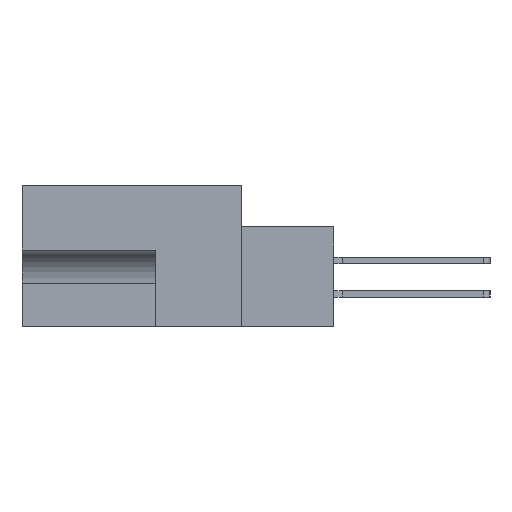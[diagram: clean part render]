
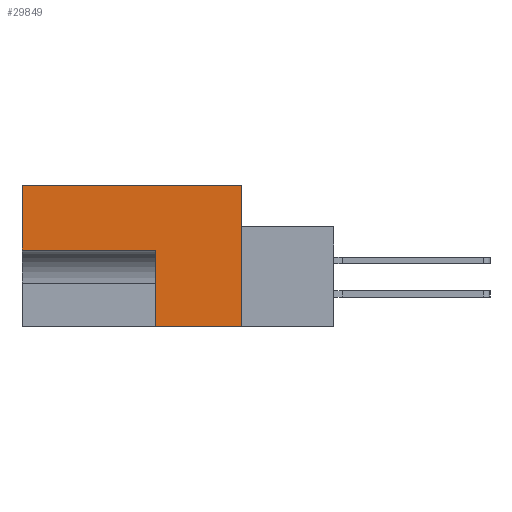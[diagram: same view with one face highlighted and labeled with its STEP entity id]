
A CAD part, left-side view. The second image highlights one B-rep face of the part: STEP entity #29849.
In plain terms, the highlighted planar face has unit normal (-1, 0, 0).
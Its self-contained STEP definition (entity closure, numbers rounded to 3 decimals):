
#51 = VERTEX_POINT ( 'NONE', #46277 ) ;
#1317 = DIRECTION ( 'NONE',  ( 1., 0., 0. ) ) ;
#1569 = ORIENTED_EDGE ( 'NONE', *, *, #10130, .F. ) ;
#1701 = DIRECTION ( 'NONE',  ( 0., 0., -1. ) ) ;
#2221 = ORIENTED_EDGE ( 'NONE', *, *, #9376, .F. ) ;
#2497 = AXIS2_PLACEMENT_3D ( 'NONE', #43975, #1317, #15414 ) ;
#2968 = VERTEX_POINT ( 'NONE', #28718 ) ;
#4047 = EDGE_CURVE ( 'NONE', #51, #22606, #5788, .T. ) ;
#5521 = EDGE_CURVE ( 'NONE', #15819, #34559, #16864, .T. ) ;
#5788 = LINE ( 'NONE', #9477, #11433 ) ;
#6238 = EDGE_LOOP ( 'NONE', ( #42021, #45216, #1569, #29505, #16491, #2221 ) ) ;
#6247 = VECTOR ( 'NONE', #1701, 1000. ) ;
#6517 = CARTESIAN_POINT ( 'NONE',  ( 0., 8.255, -13.487 ) ) ;
#7277 = FACE_OUTER_BOUND ( 'NONE', #6238, .T. ) ;
#9376 = EDGE_CURVE ( 'NONE', #30089, #51, #42847, .T. ) ;
#9457 = EDGE_CURVE ( 'NONE', #34559, #30089, #16005, .T. ) ;
#9477 = CARTESIAN_POINT ( 'NONE',  ( 0., 8.255, -6.172 ) ) ;
#9478 = CARTESIAN_POINT ( 'NONE',  ( 0., 8.255, -13.487 ) ) ;
#10130 = EDGE_CURVE ( 'NONE', #2968, #15819, #40356, .T. ) ;
#11433 = VECTOR ( 'NONE', #23053, 1000. ) ;
#12994 = VECTOR ( 'NONE', #29550, 1000. ) ;
#14346 = VECTOR ( 'NONE', #31221, 1000. ) ;
#15414 = DIRECTION ( 'NONE',  ( 0., 0., -1. ) ) ;
#15443 = VECTOR ( 'NONE', #31815, 1000. ) ;
#15819 = VERTEX_POINT ( 'NONE', #40574 ) ;
#16005 = LINE ( 'NONE', #45526, #14346 ) ;
#16491 = ORIENTED_EDGE ( 'NONE', *, *, #4047, .F. ) ;
#16864 = LINE ( 'NONE', #37464, #6247 ) ;
#17098 = LINE ( 'NONE', #27878, #15443 ) ;
#17145 = CARTESIAN_POINT ( 'NONE',  ( 0., 0., -13.487 ) ) ;
#22606 = VERTEX_POINT ( 'NONE', #33415 ) ;
#23053 = DIRECTION ( 'NONE',  ( 0., 1., 0. ) ) ;
#26087 = VECTOR ( 'NONE', #35108, 1000. ) ;
#27878 = CARTESIAN_POINT ( 'NONE',  ( 0., 20.955, -13.487 ) ) ;
#28718 = CARTESIAN_POINT ( 'NONE',  ( 0., 20.955, 0. ) ) ;
#29505 = ORIENTED_EDGE ( 'NONE', *, *, #41021, .F. ) ;
#29550 = DIRECTION ( 'NONE',  ( 0., -1., 0. ) ) ;
#29849 = ADVANCED_FACE ( 'NONE', ( #7277 ), #36809, .F. ) ;
#30089 = VERTEX_POINT ( 'NONE', #9478 ) ;
#31221 = DIRECTION ( 'NONE',  ( 0., 1., 0. ) ) ;
#31815 = DIRECTION ( 'NONE',  ( 0., 0., 1. ) ) ;
#33415 = CARTESIAN_POINT ( 'NONE',  ( 0., 20.955, -6.172 ) ) ;
#34559 = VERTEX_POINT ( 'NONE', #17145 ) ;
#35108 = DIRECTION ( 'NONE',  ( 0., 0., 1. ) ) ;
#36809 = PLANE ( 'NONE',  #2497 ) ;
#37464 = CARTESIAN_POINT ( 'NONE',  ( 0., 0., 0. ) ) ;
#40356 = LINE ( 'NONE', #43619, #12994 ) ;
#40574 = CARTESIAN_POINT ( 'NONE',  ( 0., 0., 0. ) ) ;
#41021 = EDGE_CURVE ( 'NONE', #22606, #2968, #17098, .T. ) ;
#42021 = ORIENTED_EDGE ( 'NONE', *, *, #9457, .F. ) ;
#42847 = LINE ( 'NONE', #6517, #26087 ) ;
#43619 = CARTESIAN_POINT ( 'NONE',  ( 0., 11.506, 0. ) ) ;
#43975 = CARTESIAN_POINT ( 'NONE',  ( 0., 0., 0. ) ) ;
#45216 = ORIENTED_EDGE ( 'NONE', *, *, #5521, .F. ) ;
#45526 = CARTESIAN_POINT ( 'NONE',  ( 0., -8.814, -13.487 ) ) ;
#46277 = CARTESIAN_POINT ( 'NONE',  ( 0., 8.255, -6.172 ) ) ;
